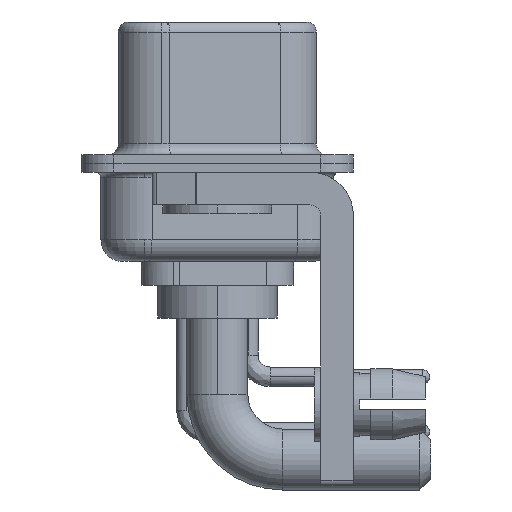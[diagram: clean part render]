
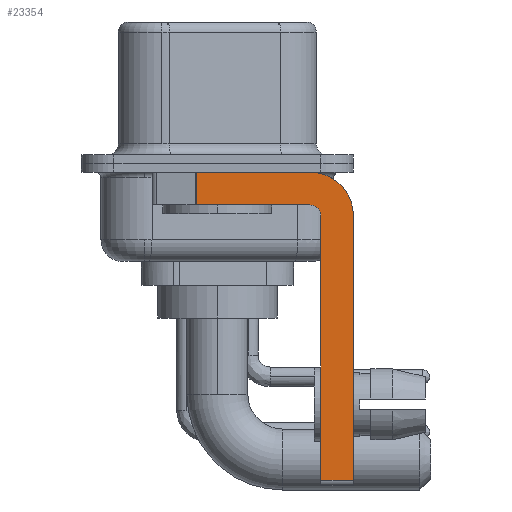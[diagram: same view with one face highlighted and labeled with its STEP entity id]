
A CAD part, left-side view. The second image highlights one B-rep face of the part: STEP entity #23354.
In plain terms, the highlighted planar face has unit normal (-1, 0, 0).
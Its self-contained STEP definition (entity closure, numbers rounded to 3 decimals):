
#24 = CARTESIAN_POINT ( 'NONE',  ( -2.9, -4.25, -2.4 ) ) ;
#700 = CARTESIAN_POINT ( 'NONE',  ( -2.9, -6.25, -2.4 ) ) ;
#795 = DIRECTION ( 'NONE',  ( 0., 0., -1. ) ) ;
#1329 = CARTESIAN_POINT ( 'NONE',  ( -2.9, -4.25, -2.4 ) ) ;
#1395 = VERTEX_POINT ( 'NONE', #7585 ) ;
#1643 = ORIENTED_EDGE ( 'NONE', *, *, #26736, .F. ) ;
#1782 = AXIS2_PLACEMENT_3D ( 'NONE', #24, #18011, #24782 ) ;
#1801 = VECTOR ( 'NONE', #1864, 1000. ) ;
#1864 = DIRECTION ( 'NONE',  ( 0., 1., 0. ) ) ;
#1889 = ORIENTED_EDGE ( 'NONE', *, *, #10754, .T. ) ;
#1988 = VERTEX_POINT ( 'NONE', #9509 ) ;
#3099 = AXIS2_PLACEMENT_3D ( 'NONE', #6319, #12791, #3818 ) ;
#3315 = EDGE_CURVE ( 'NONE', #7688, #1395, #21004, .T. ) ;
#3363 = VECTOR ( 'NONE', #12899, 1000. ) ;
#3401 = ORIENTED_EDGE ( 'NONE', *, *, #6097, .F. ) ;
#3403 = FACE_OUTER_BOUND ( 'NONE', #18405, .T. ) ;
#3808 = CARTESIAN_POINT ( 'NONE',  ( -2.9, -4.25, -1.9 ) ) ;
#3818 = DIRECTION ( 'NONE',  ( 0., 0., 1. ) ) ;
#3930 = LINE ( 'NONE', #22045, #3363 ) ;
#4747 = CARTESIAN_POINT ( 'NONE',  ( -2.9, 0.978, -1.9 ) ) ;
#5008 = LINE ( 'NONE', #3808, #1801 ) ;
#5636 = PLANE ( 'NONE',  #16728 ) ;
#5772 = DIRECTION ( 'NONE',  ( 1., 0., 0. ) ) ;
#6097 = EDGE_CURVE ( 'NONE', #22299, #1988, #23632, .T. ) ;
#6165 = CARTESIAN_POINT ( 'NONE',  ( -2.9, 3., -0.4 ) ) ;
#6319 = CARTESIAN_POINT ( 'NONE',  ( -2.9, -4.25, -2.4 ) ) ;
#6579 = VERTEX_POINT ( 'NONE', #17517 ) ;
#7585 = CARTESIAN_POINT ( 'NONE',  ( -2.9, -6.25, -14.55 ) ) ;
#7688 = VERTEX_POINT ( 'NONE', #700 ) ;
#7925 = ORIENTED_EDGE ( 'NONE', *, *, #10339, .F. ) ;
#7998 = CARTESIAN_POINT ( 'NONE',  ( -2.9, -4.75, -14.8 ) ) ;
#8581 = DIRECTION ( 'NONE',  ( 0., 0., 1. ) ) ;
#9509 = CARTESIAN_POINT ( 'NONE',  ( -2.9, -4.75, -2.4 ) ) ;
#10339 = EDGE_CURVE ( 'NONE', #1988, #21777, #17211, .T. ) ;
#10754 = EDGE_CURVE ( 'NONE', #15604, #26093, #3930, .T. ) ;
#12223 = CARTESIAN_POINT ( 'NONE',  ( -2.9, -4.25, -1.9 ) ) ;
#12554 = ORIENTED_EDGE ( 'NONE', *, *, #3315, .F. ) ;
#12643 = LINE ( 'NONE', #6165, #15143 ) ;
#12791 = DIRECTION ( 'NONE',  ( -1., 0., 0. ) ) ;
#12899 = DIRECTION ( 'NONE',  ( 0., 0., -1. ) ) ;
#13443 = LINE ( 'NONE', #16095, #15663 ) ;
#13895 = EDGE_CURVE ( 'NONE', #15604, #6579, #12643, .T. ) ;
#14026 = DIRECTION ( 'NONE',  ( 0., -1., 0. ) ) ;
#15143 = VECTOR ( 'NONE', #15152, 1000. ) ;
#15144 = EDGE_CURVE ( 'NONE', #22299, #1395, #13443, .T. ) ;
#15152 = DIRECTION ( 'NONE',  ( 0., -1., 0. ) ) ;
#15604 = VERTEX_POINT ( 'NONE', #16212 ) ;
#15663 = VECTOR ( 'NONE', #14026, 1000. ) ;
#15725 = VECTOR ( 'NONE', #8581, 1000. ) ;
#16090 = VECTOR ( 'NONE', #795, 1000. ) ;
#16095 = CARTESIAN_POINT ( 'NONE',  ( -2.9, -4.25, -14.55 ) ) ;
#16212 = CARTESIAN_POINT ( 'NONE',  ( -2.9, 0.978, -0.4 ) ) ;
#16728 = AXIS2_PLACEMENT_3D ( 'NONE', #1329, #5772, #19033 ) ;
#16857 = CIRCLE ( 'NONE', #1782, 2. ) ;
#17211 = CIRCLE ( 'NONE', #3099, 0.5 ) ;
#17517 = CARTESIAN_POINT ( 'NONE',  ( -2.9, -4.25, -0.4 ) ) ;
#18011 = DIRECTION ( 'NONE',  ( 1., 0., 0. ) ) ;
#18032 = ORIENTED_EDGE ( 'NONE', *, *, #15144, .T. ) ;
#18405 = EDGE_LOOP ( 'NONE', ( #26546, #1889, #1643, #7925, #3401, #18032, #12554, #22152 ) ) ;
#18796 = CARTESIAN_POINT ( 'NONE',  ( -2.9, -6.25, -2.4 ) ) ;
#19033 = DIRECTION ( 'NONE',  ( 0., 0., -1. ) ) ;
#21004 = LINE ( 'NONE', #18796, #16090 ) ;
#21777 = VERTEX_POINT ( 'NONE', #12223 ) ;
#22045 = CARTESIAN_POINT ( 'NONE',  ( -2.9, 0.978, -1.9 ) ) ;
#22152 = ORIENTED_EDGE ( 'NONE', *, *, #26098, .F. ) ;
#22299 = VERTEX_POINT ( 'NONE', #26780 ) ;
#23354 = ADVANCED_FACE ( 'NONE', ( #3403 ), #5636, .F. ) ;
#23632 = LINE ( 'NONE', #7998, #15725 ) ;
#24782 = DIRECTION ( 'NONE',  ( 0., 0., -1. ) ) ;
#26093 = VERTEX_POINT ( 'NONE', #4747 ) ;
#26098 = EDGE_CURVE ( 'NONE', #6579, #7688, #16857, .T. ) ;
#26546 = ORIENTED_EDGE ( 'NONE', *, *, #13895, .F. ) ;
#26736 = EDGE_CURVE ( 'NONE', #21777, #26093, #5008, .T. ) ;
#26780 = CARTESIAN_POINT ( 'NONE',  ( -2.9, -4.75, -14.55 ) ) ;
